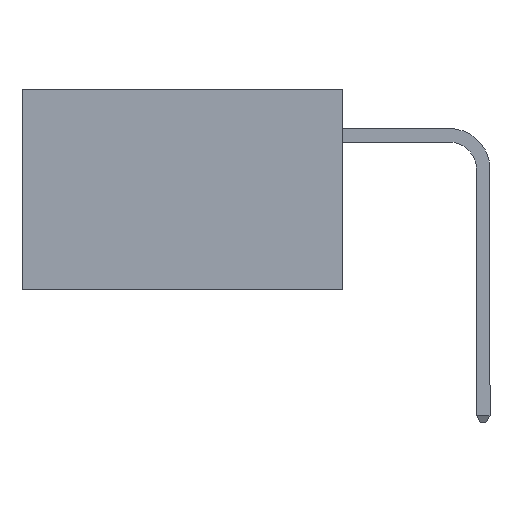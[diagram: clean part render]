
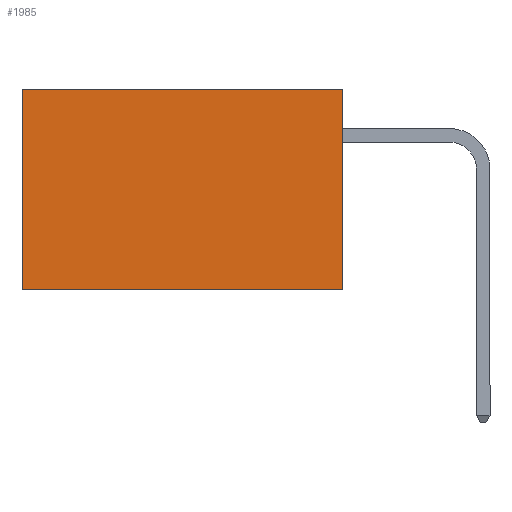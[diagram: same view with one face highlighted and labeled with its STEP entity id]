
A CAD part, left-side view. The second image highlights one B-rep face of the part: STEP entity #1985.
In plain terms, the highlighted planar face has unit normal (-1, 0, 0).
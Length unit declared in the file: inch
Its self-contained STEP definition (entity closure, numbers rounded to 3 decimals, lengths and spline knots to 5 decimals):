
#243 = LINE ( 'NONE', #5626, #4890 ) ;
#857 = CARTESIAN_POINT ( 'NONE',  ( 0.277, 0., -0.37 ) ) ;
#1327 = VERTEX_POINT ( 'NONE', #6634 ) ;
#1483 = DIRECTION ( 'NONE',  ( 0., 0., -1. ) ) ;
#1664 = FACE_OUTER_BOUND ( 'NONE', #2542, .T. ) ;
#1985 = ADVANCED_FACE ( 'NONE', ( #1664 ), #3604, .F. ) ;
#2215 = VERTEX_POINT ( 'NONE', #4132 ) ;
#2250 = LINE ( 'NONE', #4104, #5284 ) ;
#2352 = EDGE_CURVE ( 'NONE', #2215, #1327, #7258, .T. ) ;
#2459 = EDGE_CURVE ( 'NONE', #7301, #2627, #2250, .T. ) ;
#2542 = EDGE_LOOP ( 'NONE', ( #2850, #3062, #3349, #3418 ) ) ;
#2580 = CARTESIAN_POINT ( 'NONE',  ( 0.277, 0.59, -0.37 ) ) ;
#2627 = VERTEX_POINT ( 'NONE', #2580 ) ;
#2697 = CARTESIAN_POINT ( 'NONE',  ( 0.277, 0., 0. ) ) ;
#2850 = ORIENTED_EDGE ( 'NONE', *, *, #4028, .T. ) ;
#3062 = ORIENTED_EDGE ( 'NONE', *, *, #2459, .F. ) ;
#3349 = ORIENTED_EDGE ( 'NONE', *, *, #7355, .F. ) ;
#3418 = ORIENTED_EDGE ( 'NONE', *, *, #2352, .T. ) ;
#3554 = DIRECTION ( 'NONE',  ( 1., 0., 0. ) ) ;
#3604 = PLANE ( 'NONE',  #6007 ) ;
#3621 = CARTESIAN_POINT ( 'NONE',  ( 0.277, 0., -0.37 ) ) ;
#4028 = EDGE_CURVE ( 'NONE', #1327, #2627, #243, .T. ) ;
#4104 = CARTESIAN_POINT ( 'NONE',  ( 0.277, 0., -0.37 ) ) ;
#4106 = DIRECTION ( 'NONE',  ( 0., 0., -1. ) ) ;
#4132 = CARTESIAN_POINT ( 'NONE',  ( 0.277, 0., 0. ) ) ;
#4171 = VECTOR ( 'NONE', #1483, 39.37008 ) ;
#4890 = VECTOR ( 'NONE', #5081, 39.37008 ) ;
#5081 = DIRECTION ( 'NONE',  ( 0., 0., -1. ) ) ;
#5284 = VECTOR ( 'NONE', #7270, 39.37008 ) ;
#5522 = LINE ( 'NONE', #6683, #4171 ) ;
#5626 = CARTESIAN_POINT ( 'NONE',  ( 0.277, 0.59, -0.37 ) ) ;
#6007 = AXIS2_PLACEMENT_3D ( 'NONE', #3621, #3554, #4106 ) ;
#6108 = DIRECTION ( 'NONE',  ( 0., 1., 0. ) ) ;
#6634 = CARTESIAN_POINT ( 'NONE',  ( 0.277, 0.59, 0. ) ) ;
#6683 = CARTESIAN_POINT ( 'NONE',  ( 0.277, 0., -0.37 ) ) ;
#7086 = VECTOR ( 'NONE', #6108, 39.37008 ) ;
#7258 = LINE ( 'NONE', #2697, #7086 ) ;
#7270 = DIRECTION ( 'NONE',  ( 0., 1., 0. ) ) ;
#7301 = VERTEX_POINT ( 'NONE', #857 ) ;
#7355 = EDGE_CURVE ( 'NONE', #2215, #7301, #5522, .T. ) ;
